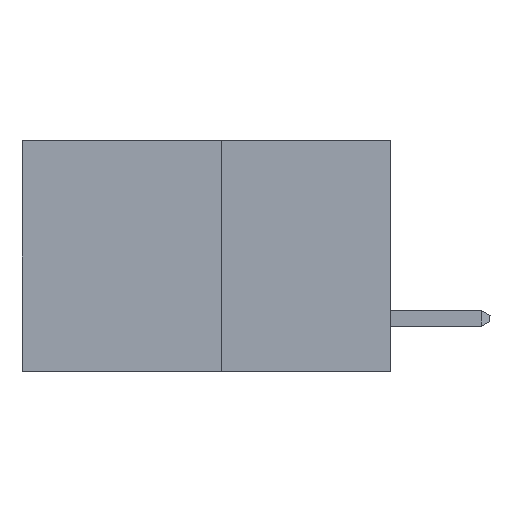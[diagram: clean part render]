
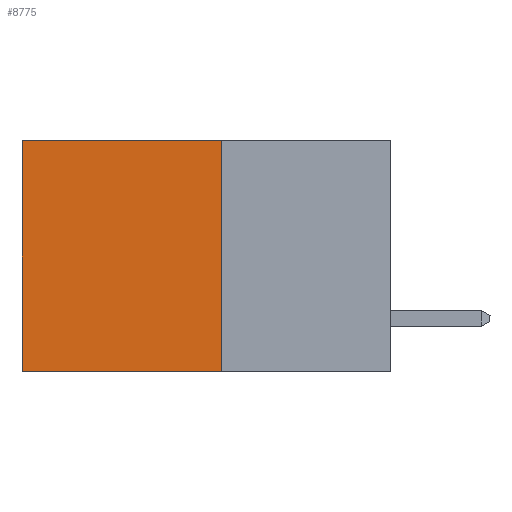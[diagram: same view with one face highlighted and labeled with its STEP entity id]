
A CAD part, left-side view. The second image highlights one B-rep face of the part: STEP entity #8775.
In plain terms, the highlighted planar face has unit normal (-1, 0, 0).
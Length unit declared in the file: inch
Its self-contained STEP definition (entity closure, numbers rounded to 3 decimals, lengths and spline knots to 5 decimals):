
#143 = VERTEX_POINT ( 'NONE', #11638 ) ;
#350 = FACE_OUTER_BOUND ( 'NONE', #7503, .T. ) ;
#351 = VERTEX_POINT ( 'NONE', #3574 ) ;
#380 = DIRECTION ( 'NONE',  ( 0., 0., -1. ) ) ;
#954 = EDGE_CURVE ( 'NONE', #3965, #351, #4471, .T. ) ;
#1025 = DIRECTION ( 'NONE',  ( 0., 0., -1. ) ) ;
#1093 = VECTOR ( 'NONE', #2384, 39.37008 ) ;
#1499 = CARTESIAN_POINT ( 'NONE',  ( 0.277, 0.27, 0. ) ) ;
#1996 = VECTOR ( 'NONE', #4453, 39.37008 ) ;
#2060 = VECTOR ( 'NONE', #8239, 39.37008 ) ;
#2216 = VERTEX_POINT ( 'NONE', #7519 ) ;
#2384 = DIRECTION ( 'NONE',  ( 0., 1., 0. ) ) ;
#3160 = CARTESIAN_POINT ( 'NONE',  ( 0.277, 0.27, -0.37 ) ) ;
#3574 = CARTESIAN_POINT ( 'NONE',  ( 0.277, 0.59, -0.37 ) ) ;
#3965 = VERTEX_POINT ( 'NONE', #6471 ) ;
#4453 = DIRECTION ( 'NONE',  ( 0., 0., -1. ) ) ;
#4471 = LINE ( 'NONE', #5233, #2060 ) ;
#4996 = PLANE ( 'NONE',  #8180 ) ;
#5233 = CARTESIAN_POINT ( 'NONE',  ( 0.277, 0.27, -0.37 ) ) ;
#5894 = DIRECTION ( 'NONE',  ( 1., 0., 0. ) ) ;
#6240 = CARTESIAN_POINT ( 'NONE',  ( 0.277, 0.59, -0.37 ) ) ;
#6471 = CARTESIAN_POINT ( 'NONE',  ( 0.277, 0.27, -0.37 ) ) ;
#7363 = EDGE_CURVE ( 'NONE', #143, #351, #9220, .T. ) ;
#7411 = CARTESIAN_POINT ( 'NONE',  ( 0.277, 0.27, -0.37 ) ) ;
#7503 = EDGE_LOOP ( 'NONE', ( #8083, #10398, #8367, #8649 ) ) ;
#7519 = CARTESIAN_POINT ( 'NONE',  ( 0.277, 0.27, 0. ) ) ;
#8083 = ORIENTED_EDGE ( 'NONE', *, *, #7363, .T. ) ;
#8180 = AXIS2_PLACEMENT_3D ( 'NONE', #3160, #5894, #380 ) ;
#8212 = EDGE_CURVE ( 'NONE', #2216, #3965, #11106, .T. ) ;
#8239 = DIRECTION ( 'NONE',  ( 0., 1., 0. ) ) ;
#8367 = ORIENTED_EDGE ( 'NONE', *, *, #8212, .F. ) ;
#8389 = LINE ( 'NONE', #1499, #1093 ) ;
#8649 = ORIENTED_EDGE ( 'NONE', *, *, #9935, .T. ) ;
#8775 = ADVANCED_FACE ( 'NONE', ( #350 ), #4996, .F. ) ;
#8833 = VECTOR ( 'NONE', #1025, 39.37008 ) ;
#9220 = LINE ( 'NONE', #6240, #1996 ) ;
#9935 = EDGE_CURVE ( 'NONE', #2216, #143, #8389, .T. ) ;
#10398 = ORIENTED_EDGE ( 'NONE', *, *, #954, .F. ) ;
#11106 = LINE ( 'NONE', #7411, #8833 ) ;
#11638 = CARTESIAN_POINT ( 'NONE',  ( 0.277, 0.59, 0. ) ) ;
